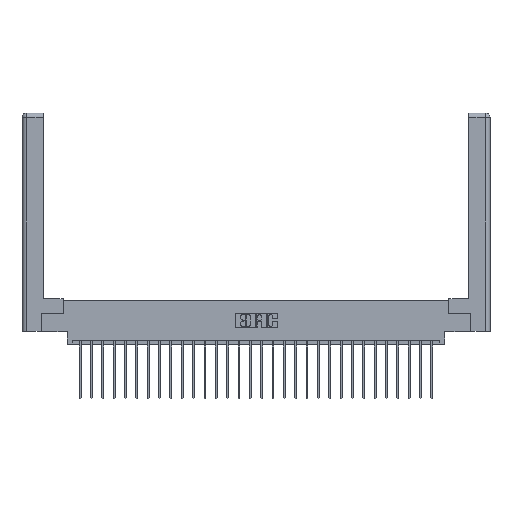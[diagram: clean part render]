
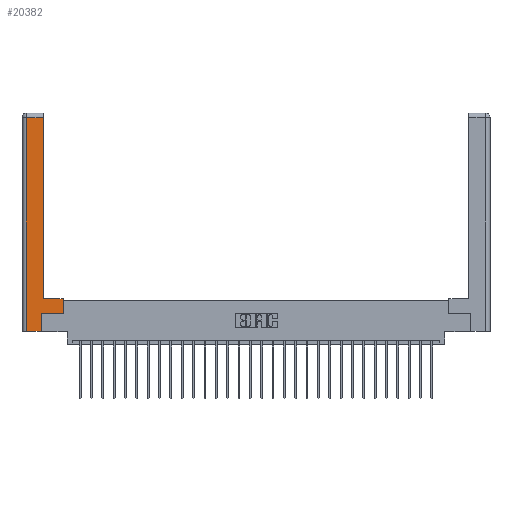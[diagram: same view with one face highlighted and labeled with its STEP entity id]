
A CAD part, top view. The second image highlights one B-rep face of the part: STEP entity #20382.
In plain terms, the highlighted planar face has unit normal (0, 0, 1).
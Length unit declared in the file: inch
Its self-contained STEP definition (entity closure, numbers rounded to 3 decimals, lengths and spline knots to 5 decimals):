
#424 = CARTESIAN_POINT ( 'NONE',  ( 0.565, 0.45, 0. ) ) ;
#562 = EDGE_CURVE ( 'NONE', #1969, #5017, #23113, .T. ) ;
#900 = DIRECTION ( 'NONE',  ( 0., 1., 0. ) ) ;
#1341 = VECTOR ( 'NONE', #15206, 39.37008 ) ;
#1969 = VERTEX_POINT ( 'NONE', #28226 ) ;
#2899 = ORIENTED_EDGE ( 'NONE', *, *, #27616, .T. ) ;
#5017 = VERTEX_POINT ( 'NONE', #27606 ) ;
#5090 = CARTESIAN_POINT ( 'NONE',  ( 0.0615, 2.94, 0. ) ) ;
#6859 = LINE ( 'NONE', #21954, #15579 ) ;
#7280 = VECTOR ( 'NONE', #900, 39.37008 ) ;
#7653 = ORIENTED_EDGE ( 'NONE', *, *, #20700, .T. ) ;
#8415 = FACE_OUTER_BOUND ( 'NONE', #28743, .T. ) ;
#8675 = PLANE ( 'NONE',  #11766 ) ;
#9081 = EDGE_CURVE ( 'NONE', #16857, #28722, #23478, .T. ) ;
#10041 = VECTOR ( 'NONE', #16271, 39.37008 ) ;
#10361 = CARTESIAN_POINT ( 'NONE',  ( 0.0615, 0., 0. ) ) ;
#11216 = DIRECTION ( 'NONE',  ( 0., -1., 0. ) ) ;
#11345 = ORIENTED_EDGE ( 'NONE', *, *, #27303, .T. ) ;
#11766 = AXIS2_PLACEMENT_3D ( 'NONE', #28670, #19383, #12842 ) ;
#12011 = VECTOR ( 'NONE', #19523, 39.37008 ) ;
#12439 = CARTESIAN_POINT ( 'NONE',  ( 0.265, 0.245, 0. ) ) ;
#12706 = EDGE_CURVE ( 'NONE', #5017, #21683, #20414, .T. ) ;
#12842 = DIRECTION ( 'NONE',  ( -1., 0., 0. ) ) ;
#13593 = VERTEX_POINT ( 'NONE', #23800 ) ;
#13702 = EDGE_CURVE ( 'NONE', #28722, #21520, #6859, .T. ) ;
#14284 = ORIENTED_EDGE ( 'NONE', *, *, #13702, .T. ) ;
#15148 = ORIENTED_EDGE ( 'NONE', *, *, #12706, .T. ) ;
#15206 = DIRECTION ( 'NONE',  ( 0., 1., 0. ) ) ;
#15579 = VECTOR ( 'NONE', #21844, 39.37008 ) ;
#15636 = LINE ( 'NONE', #25260, #7280 ) ;
#16024 = DIRECTION ( 'NONE',  ( 1., 0., 0. ) ) ;
#16271 = DIRECTION ( 'NONE',  ( -1., 0., 0. ) ) ;
#16450 = VERTEX_POINT ( 'NONE', #12439 ) ;
#16460 = VECTOR ( 'NONE', #11216, 39.37008 ) ;
#16857 = VERTEX_POINT ( 'NONE', #27526 ) ;
#17151 = CARTESIAN_POINT ( 'NONE',  ( 0.265, 0.245, 0. ) ) ;
#17501 = VECTOR ( 'NONE', #27252, 39.37008 ) ;
#18465 = CARTESIAN_POINT ( 'NONE',  ( 0.565, 0.245, 0. ) ) ;
#19383 = DIRECTION ( 'NONE',  ( 0., 0., -1. ) ) ;
#19523 = DIRECTION ( 'NONE',  ( -1., 0., 0. ) ) ;
#19700 = EDGE_CURVE ( 'NONE', #13593, #16857, #25747, .T. ) ;
#20111 = CARTESIAN_POINT ( 'NONE',  ( 0.0615, 0., 0. ) ) ;
#20382 = ADVANCED_FACE ( 'NONE', ( #8415 ), #8675, .F. ) ;
#20414 = LINE ( 'NONE', #26441, #12011 ) ;
#20700 = EDGE_CURVE ( 'NONE', #16450, #1969, #28629, .T. ) ;
#21520 = VERTEX_POINT ( 'NONE', #25546 ) ;
#21683 = VERTEX_POINT ( 'NONE', #25845 ) ;
#21844 = DIRECTION ( 'NONE',  ( 1., 0., 0. ) ) ;
#21954 = CARTESIAN_POINT ( 'NONE',  ( 0.265, 0., 0. ) ) ;
#23113 = LINE ( 'NONE', #424, #17501 ) ;
#23371 = ORIENTED_EDGE ( 'NONE', *, *, #562, .T. ) ;
#23478 = LINE ( 'NONE', #10361, #16460 ) ;
#23800 = CARTESIAN_POINT ( 'NONE',  ( 0.295, 2.94, 0. ) ) ;
#24181 = ORIENTED_EDGE ( 'NONE', *, *, #9081, .T. ) ;
#24780 = VECTOR ( 'NONE', #16024, 39.37008 ) ;
#25260 = CARTESIAN_POINT ( 'NONE',  ( 0.295, 3., 0. ) ) ;
#25546 = CARTESIAN_POINT ( 'NONE',  ( 0.265, 0., 0. ) ) ;
#25747 = LINE ( 'NONE', #5090, #10041 ) ;
#25845 = CARTESIAN_POINT ( 'NONE',  ( 0.295, 0.45, 0. ) ) ;
#26301 = ORIENTED_EDGE ( 'NONE', *, *, #19700, .T. ) ;
#26441 = CARTESIAN_POINT ( 'NONE',  ( 0.295, 0.45, 0. ) ) ;
#26455 = LINE ( 'NONE', #17151, #1341 ) ;
#27252 = DIRECTION ( 'NONE',  ( 0., 1., 0. ) ) ;
#27303 = EDGE_CURVE ( 'NONE', #21683, #13593, #15636, .T. ) ;
#27526 = CARTESIAN_POINT ( 'NONE',  ( 0.0615, 2.94, 0. ) ) ;
#27606 = CARTESIAN_POINT ( 'NONE',  ( 0.565, 0.45, 0. ) ) ;
#27616 = EDGE_CURVE ( 'NONE', #21520, #16450, #26455, .T. ) ;
#28226 = CARTESIAN_POINT ( 'NONE',  ( 0.565, 0.245, 0. ) ) ;
#28629 = LINE ( 'NONE', #18465, #24780 ) ;
#28670 = CARTESIAN_POINT ( 'NONE',  ( 0., 0., 0. ) ) ;
#28722 = VERTEX_POINT ( 'NONE', #20111 ) ;
#28743 = EDGE_LOOP ( 'NONE', ( #11345, #26301, #24181, #14284, #2899, #7653, #23371, #15148 ) ) ;
